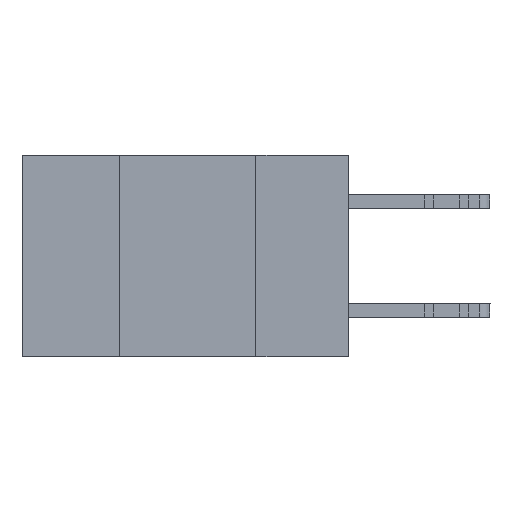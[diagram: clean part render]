
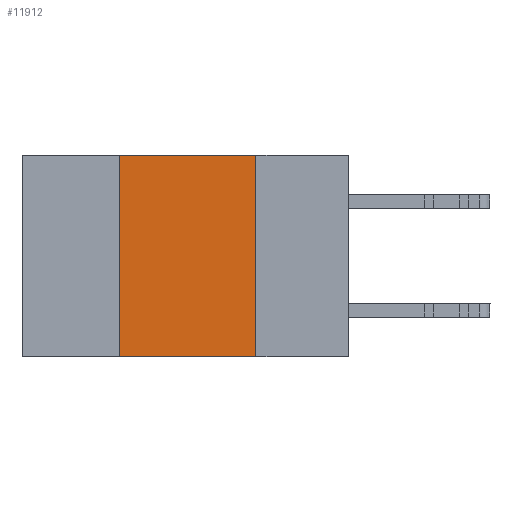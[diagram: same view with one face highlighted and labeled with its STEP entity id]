
A CAD part, left-side view. The second image highlights one B-rep face of the part: STEP entity #11912.
In plain terms, the highlighted planar face has unit normal (-1, 0, 0).
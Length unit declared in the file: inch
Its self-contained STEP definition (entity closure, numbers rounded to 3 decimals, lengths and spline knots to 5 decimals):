
#329 = EDGE_LOOP ( 'NONE', ( #485, #1803, #4952, #6978 ) ) ;
#439 = CARTESIAN_POINT ( 'NONE',  ( 0., 0.42, -0.37 ) ) ;
#485 = ORIENTED_EDGE ( 'NONE', *, *, #4885, .F. ) ;
#1033 = DIRECTION ( 'NONE',  ( 0., -1., 0. ) ) ;
#1768 = VERTEX_POINT ( 'NONE', #21676 ) ;
#1803 = ORIENTED_EDGE ( 'NONE', *, *, #14771, .F. ) ;
#1838 = DIRECTION ( 'NONE',  ( 0., -1., 0. ) ) ;
#3016 = VERTEX_POINT ( 'NONE', #12081 ) ;
#3475 = CARTESIAN_POINT ( 'NONE',  ( 0., 0.17, -0.37 ) ) ;
#3809 = CARTESIAN_POINT ( 'NONE',  ( 0., 0.6, -0.37 ) ) ;
#4344 = AXIS2_PLACEMENT_3D ( 'NONE', #4790, #18449, #6768 ) ;
#4431 = DIRECTION ( 'NONE',  ( 0., 0., 1. ) ) ;
#4790 = CARTESIAN_POINT ( 'NONE',  ( 0., 0.6, 0. ) ) ;
#4885 = EDGE_CURVE ( 'NONE', #3016, #9667, #14186, .T. ) ;
#4952 = ORIENTED_EDGE ( 'NONE', *, *, #6386, .F. ) ;
#5279 = VECTOR ( 'NONE', #1838, 39.37008 ) ;
#6386 = EDGE_CURVE ( 'NONE', #1768, #17635, #15011, .T. ) ;
#6768 = DIRECTION ( 'NONE',  ( 0., 0., -1. ) ) ;
#6978 = ORIENTED_EDGE ( 'NONE', *, *, #19958, .T. ) ;
#9640 = VECTOR ( 'NONE', #11326, 39.37008 ) ;
#9667 = VERTEX_POINT ( 'NONE', #17607 ) ;
#9871 = VECTOR ( 'NONE', #4431, 39.37008 ) ;
#11326 = DIRECTION ( 'NONE',  ( 0., 0., -1. ) ) ;
#11696 = LINE ( 'NONE', #12838, #22560 ) ;
#11912 = ADVANCED_FACE ( 'NONE', ( #20327 ), #12613, .F. ) ;
#12081 = CARTESIAN_POINT ( 'NONE',  ( 0., 0.17, 0. ) ) ;
#12613 = PLANE ( 'NONE',  #4344 ) ;
#12740 = CARTESIAN_POINT ( 'NONE',  ( 0., 0.42, 0. ) ) ;
#12838 = CARTESIAN_POINT ( 'NONE',  ( 0., 0.6, 0. ) ) ;
#14186 = LINE ( 'NONE', #3475, #9640 ) ;
#14771 = EDGE_CURVE ( 'NONE', #17635, #3016, #11696, .T. ) ;
#15011 = LINE ( 'NONE', #439, #9871 ) ;
#17607 = CARTESIAN_POINT ( 'NONE',  ( 0., 0.17, -0.37 ) ) ;
#17635 = VERTEX_POINT ( 'NONE', #12740 ) ;
#18449 = DIRECTION ( 'NONE',  ( 1., 0., 0. ) ) ;
#19958 = EDGE_CURVE ( 'NONE', #1768, #9667, #20816, .T. ) ;
#20327 = FACE_OUTER_BOUND ( 'NONE', #329, .T. ) ;
#20816 = LINE ( 'NONE', #3809, #5279 ) ;
#21676 = CARTESIAN_POINT ( 'NONE',  ( 0., 0.42, -0.37 ) ) ;
#22560 = VECTOR ( 'NONE', #1033, 39.37008 ) ;
